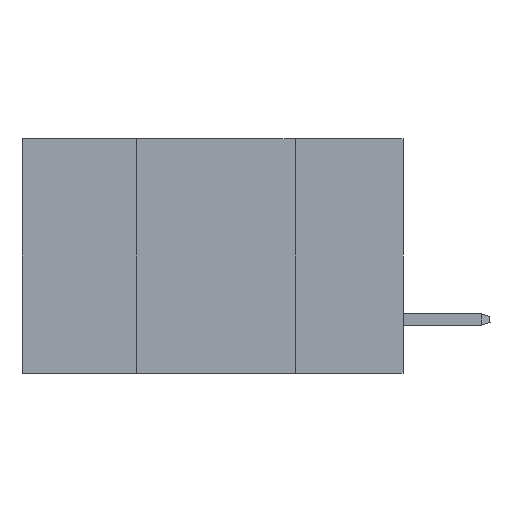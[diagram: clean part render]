
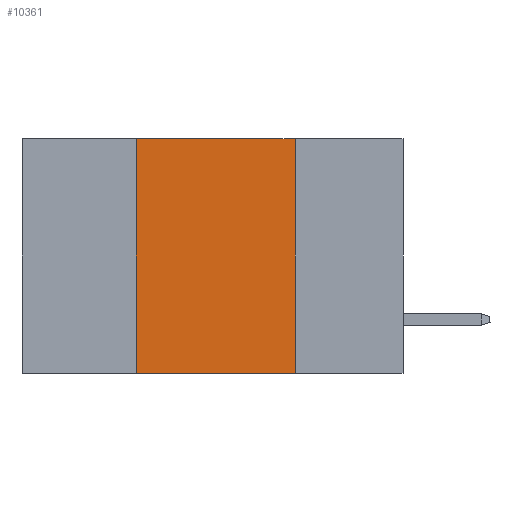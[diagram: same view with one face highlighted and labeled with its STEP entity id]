
A CAD part, left-side view. The second image highlights one B-rep face of the part: STEP entity #10361.
In plain terms, the highlighted planar face has unit normal (-1, 0, 0).
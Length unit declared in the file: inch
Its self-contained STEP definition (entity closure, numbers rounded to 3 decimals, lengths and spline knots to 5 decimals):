
#2092 = ORIENTED_EDGE ( 'NONE', *, *, #18245, .F. ) ;
#2268 = EDGE_CURVE ( 'NONE', #15823, #3086, #5052, .T. ) ;
#2295 = AXIS2_PLACEMENT_3D ( 'NONE', #5029, #4740, #3183 ) ;
#3086 = VERTEX_POINT ( 'NONE', #16585 ) ;
#3183 = DIRECTION ( 'NONE',  ( 0., 0., -1. ) ) ;
#4740 = DIRECTION ( 'NONE',  ( 1., 0., 0. ) ) ;
#4881 = ORIENTED_EDGE ( 'NONE', *, *, #2268, .F. ) ;
#5011 = CARTESIAN_POINT ( 'NONE',  ( 0., 0.17, 0. ) ) ;
#5029 = CARTESIAN_POINT ( 'NONE',  ( 0., 0.6, 0. ) ) ;
#5052 = LINE ( 'NONE', #8312, #12259 ) ;
#5302 = LINE ( 'NONE', #5011, #13607 ) ;
#5697 = EDGE_CURVE ( 'NONE', #10197, #11620, #5302, .T. ) ;
#6540 = DIRECTION ( 'NONE',  ( 0., 0., 1. ) ) ;
#7414 = EDGE_CURVE ( 'NONE', #15823, #11620, #11955, .T. ) ;
#8312 = CARTESIAN_POINT ( 'NONE',  ( 0., 0.42, 0. ) ) ;
#8697 = CARTESIAN_POINT ( 'NONE',  ( 0., 0.17, 0. ) ) ;
#9576 = PLANE ( 'NONE',  #2295 ) ;
#10197 = VERTEX_POINT ( 'NONE', #8697 ) ;
#10361 = ADVANCED_FACE ( 'NONE', ( #12232 ), #9576, .F. ) ;
#11237 = ORIENTED_EDGE ( 'NONE', *, *, #5697, .F. ) ;
#11311 = LINE ( 'NONE', #18391, #18413 ) ;
#11620 = VERTEX_POINT ( 'NONE', #15414 ) ;
#11955 = LINE ( 'NONE', #16461, #17261 ) ;
#12186 = ORIENTED_EDGE ( 'NONE', *, *, #7414, .T. ) ;
#12232 = FACE_OUTER_BOUND ( 'NONE', #16562, .T. ) ;
#12259 = VECTOR ( 'NONE', #6540, 39.37008 ) ;
#13607 = VECTOR ( 'NONE', #14087, 39.37008 ) ;
#14087 = DIRECTION ( 'NONE',  ( 0., 0., -1. ) ) ;
#14632 = CARTESIAN_POINT ( 'NONE',  ( 0., 0.42, -0.37 ) ) ;
#15414 = CARTESIAN_POINT ( 'NONE',  ( 0., 0.17, -0.37 ) ) ;
#15823 = VERTEX_POINT ( 'NONE', #14632 ) ;
#16461 = CARTESIAN_POINT ( 'NONE',  ( 0., 0.6, -0.37 ) ) ;
#16562 = EDGE_LOOP ( 'NONE', ( #11237, #2092, #4881, #12186 ) ) ;
#16585 = CARTESIAN_POINT ( 'NONE',  ( 0., 0.42, 0. ) ) ;
#17261 = VECTOR ( 'NONE', #17639, 39.37008 ) ;
#17639 = DIRECTION ( 'NONE',  ( 0., -1., 0. ) ) ;
#18245 = EDGE_CURVE ( 'NONE', #3086, #10197, #11311, .T. ) ;
#18391 = CARTESIAN_POINT ( 'NONE',  ( 0., 0.6, 0. ) ) ;
#18413 = VECTOR ( 'NONE', #18490, 39.37008 ) ;
#18490 = DIRECTION ( 'NONE',  ( 0., -1., 0. ) ) ;
